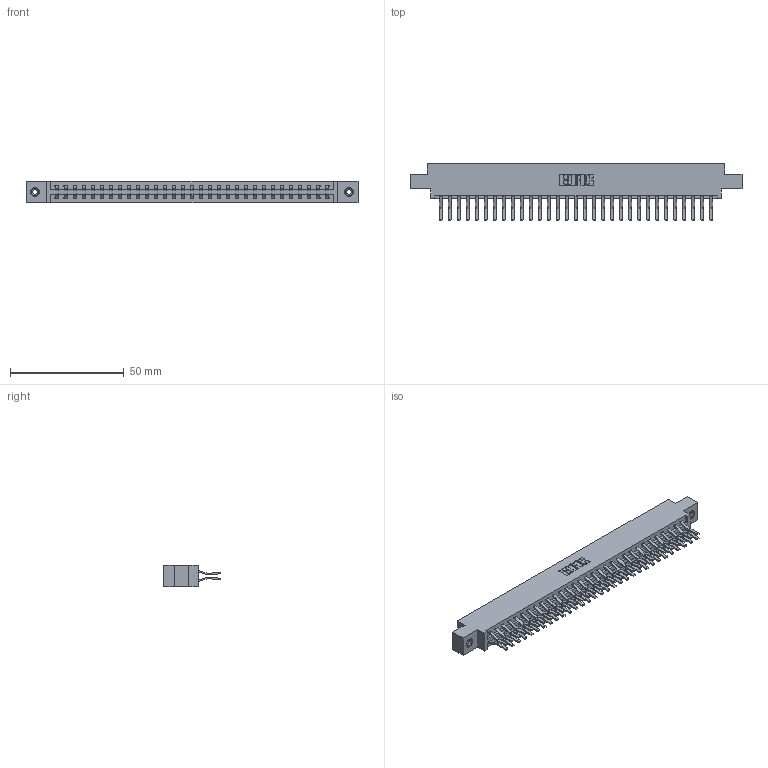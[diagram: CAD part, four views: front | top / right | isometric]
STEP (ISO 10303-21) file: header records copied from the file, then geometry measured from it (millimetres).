
FILE_DESCRIPTION (( 'STEP AP203' ), '1' );
FILE_NAME ('337-062-560-808.STEP', '2018-08-11T05:08:50', ( '' ), ( '' ), 'SwSTEP 2.0', 'SolidWorks 2016', '' );
FILE_SCHEMA (( 'CONFIG_CONTROL_DESIGN' ));
Length unit declared in the file: inch
Products named in the file (4): 345-250-001_345-250-003-102; 337-062-560-808; 337 Part_0.170 Offset - 0.156 Dia-TI; 345-292-001_560 Tail
Assembly tree (65 placements, depth 2):
  337-062-560-808
    337 Part_0.170 Offset - 0.156 Dia-TI
    345-292-001_560 Tail  x62
    345-250-001_345-250-003-102  x2
Bounding box: 145.85 x 24.78 x 9.4 mm (x, y, z)
Volume: 15506.4 mm3; surface area: 18731.1 mm2
Topology: 65 solids, 65 shells, 3650 faces, 10813 edges, 7118 vertices
Faces by surface type: plane 2462, cylinder 1172, cone 12, torus 4
Entity records: 26864 total; most frequent: CARTESIAN_POINT 4517, ORIENTED_EDGE 4446, DIRECTION 3897, EDGE_CURVE 2223, LINE 2071, VECTOR 2071, VERTEX_POINT 1476, AXIS2_PLACEMENT_3D 913
